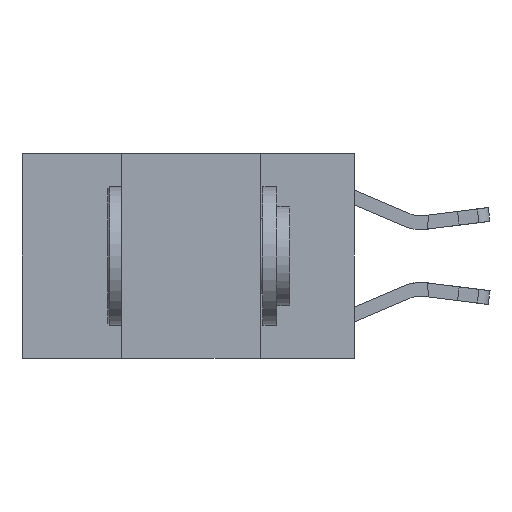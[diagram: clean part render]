
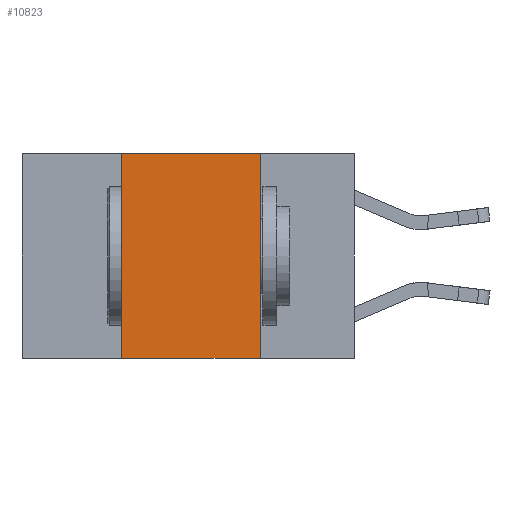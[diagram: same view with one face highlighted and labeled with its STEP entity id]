
A CAD part, left-side view. The second image highlights one B-rep face of the part: STEP entity #10823.
In plain terms, the highlighted planar face has unit normal (-1, 0, 0).
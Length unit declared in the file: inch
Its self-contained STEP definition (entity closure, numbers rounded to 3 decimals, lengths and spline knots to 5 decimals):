
#779 = VECTOR ( 'NONE', #14089, 39.37008 ) ;
#1300 = DIRECTION ( 'NONE',  ( 0., 0., 1. ) ) ;
#1872 = VECTOR ( 'NONE', #1300, 39.37008 ) ;
#1926 = LINE ( 'NONE', #13155, #19197 ) ;
#2034 = DIRECTION ( 'NONE',  ( 0., -1., 0. ) ) ;
#2109 = CARTESIAN_POINT ( 'NONE',  ( 0., 0.6, 0. ) ) ;
#2413 = ORIENTED_EDGE ( 'NONE', *, *, #13406, .F. ) ;
#2662 = LINE ( 'NONE', #15924, #779 ) ;
#3844 = DIRECTION ( 'NONE',  ( 1., 0., 0. ) ) ;
#4062 = DIRECTION ( 'NONE',  ( 0., 0., -1. ) ) ;
#4116 = LINE ( 'NONE', #20627, #1872 ) ;
#5620 = VECTOR ( 'NONE', #8825, 39.37008 ) ;
#6964 = VERTEX_POINT ( 'NONE', #18515 ) ;
#7693 = AXIS2_PLACEMENT_3D ( 'NONE', #2109, #3844, #4062 ) ;
#8825 = DIRECTION ( 'NONE',  ( 0., -1., 0. ) ) ;
#10823 = ADVANCED_FACE ( 'NONE', ( #16883 ), #15598, .F. ) ;
#12447 = VERTEX_POINT ( 'NONE', #13208 ) ;
#12604 = ORIENTED_EDGE ( 'NONE', *, *, #14065, .F. ) ;
#13155 = CARTESIAN_POINT ( 'NONE',  ( 0., 0.6, -0.37 ) ) ;
#13208 = CARTESIAN_POINT ( 'NONE',  ( 0., 0.17, -0.37 ) ) ;
#13406 = EDGE_CURVE ( 'NONE', #17418, #6964, #4116, .T. ) ;
#14065 = EDGE_CURVE ( 'NONE', #6964, #17506, #15085, .T. ) ;
#14089 = DIRECTION ( 'NONE',  ( 0., 0., -1. ) ) ;
#14202 = EDGE_CURVE ( 'NONE', #17506, #12447, #2662, .T. ) ;
#15085 = LINE ( 'NONE', #16581, #5620 ) ;
#15598 = PLANE ( 'NONE',  #7693 ) ;
#15826 = ORIENTED_EDGE ( 'NONE', *, *, #19622, .T. ) ;
#15905 = CARTESIAN_POINT ( 'NONE',  ( 0., 0.42, -0.37 ) ) ;
#15924 = CARTESIAN_POINT ( 'NONE',  ( 0., 0.17, 0. ) ) ;
#16024 = EDGE_LOOP ( 'NONE', ( #19593, #12604, #2413, #15826 ) ) ;
#16581 = CARTESIAN_POINT ( 'NONE',  ( 0., 0.6, 0. ) ) ;
#16883 = FACE_OUTER_BOUND ( 'NONE', #16024, .T. ) ;
#17418 = VERTEX_POINT ( 'NONE', #15905 ) ;
#17506 = VERTEX_POINT ( 'NONE', #19503 ) ;
#18515 = CARTESIAN_POINT ( 'NONE',  ( 0., 0.42, 0. ) ) ;
#19197 = VECTOR ( 'NONE', #2034, 39.37008 ) ;
#19503 = CARTESIAN_POINT ( 'NONE',  ( 0., 0.17, 0. ) ) ;
#19593 = ORIENTED_EDGE ( 'NONE', *, *, #14202, .F. ) ;
#19622 = EDGE_CURVE ( 'NONE', #17418, #12447, #1926, .T. ) ;
#20627 = CARTESIAN_POINT ( 'NONE',  ( 0., 0.42, 0. ) ) ;
